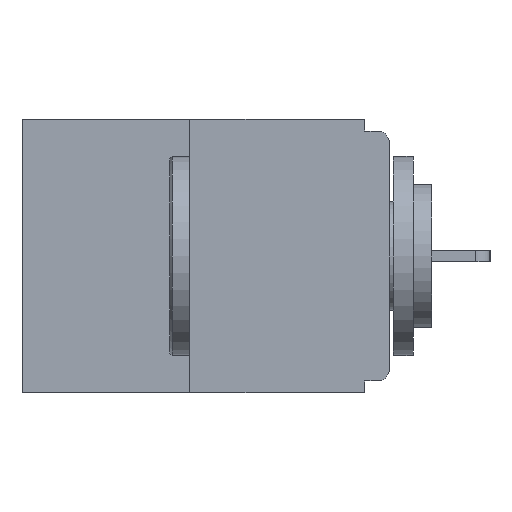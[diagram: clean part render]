
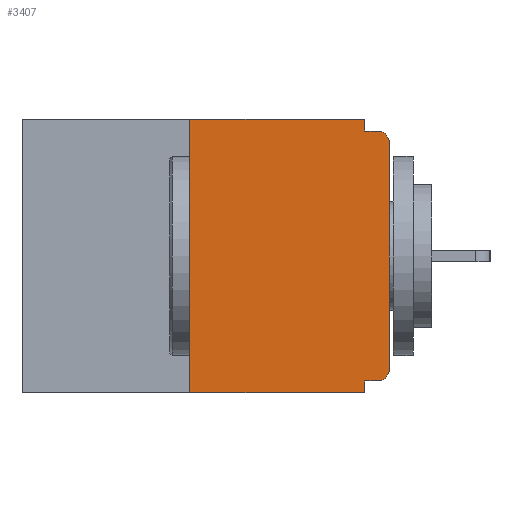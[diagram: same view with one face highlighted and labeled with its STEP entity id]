
A CAD part, left-side view. The second image highlights one B-rep face of the part: STEP entity #3407.
In plain terms, the highlighted planar face has unit normal (-1, 0, 0).
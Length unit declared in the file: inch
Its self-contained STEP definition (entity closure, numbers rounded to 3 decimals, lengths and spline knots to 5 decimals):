
#260 = VERTEX_POINT ( 'NONE', #3799 ) ;
#316 = CARTESIAN_POINT ( 'NONE',  ( 0., 0., 0. ) ) ;
#791 = AXIS2_PLACEMENT_3D ( 'NONE', #11645, #15916, #11462 ) ;
#818 = CARTESIAN_POINT ( 'NONE',  ( 0., 0., -0.03 ) ) ;
#1094 = LINE ( 'NONE', #6852, #12949 ) ;
#1300 = CARTESIAN_POINT ( 'NONE',  ( 0., 0.46, 0. ) ) ;
#1561 = DIRECTION ( 'NONE',  ( 0., 1., 0. ) ) ;
#1620 = VERTEX_POINT ( 'NONE', #3096 ) ;
#1744 = ORIENTED_EDGE ( 'NONE', *, *, #5236, .F. ) ;
#1764 = EDGE_CURVE ( 'NONE', #12057, #2645, #15228, .T. ) ;
#1953 = CARTESIAN_POINT ( 'NONE',  ( 0., 0.031, -0.328 ) ) ;
#2507 = VECTOR ( 'NONE', #6049, 39.37008 ) ;
#2645 = VERTEX_POINT ( 'NONE', #7402 ) ;
#3096 = CARTESIAN_POINT ( 'NONE',  ( 0., 0.25, -0.343 ) ) ;
#3197 = CIRCLE ( 'NONE', #6806, 0.015 ) ;
#3407 = ADVANCED_FACE ( 'NONE', ( #15350 ), #7149, .F. ) ;
#3560 = DIRECTION ( 'NONE',  ( 0., -1., 0. ) ) ;
#3799 = CARTESIAN_POINT ( 'NONE',  ( 0., 0.015, -0.328 ) ) ;
#3815 = AXIS2_PLACEMENT_3D ( 'NONE', #1300, #11373, #11275 ) ;
#3938 = VECTOR ( 'NONE', #10862, 39.37008 ) ;
#4497 = LINE ( 'NONE', #15814, #15665 ) ;
#4997 = ORIENTED_EDGE ( 'NONE', *, *, #9767, .T. ) ;
#5148 = CARTESIAN_POINT ( 'NONE',  ( 0., 0., -0.015 ) ) ;
#5236 = EDGE_CURVE ( 'NONE', #14864, #13512, #17326, .T. ) ;
#5780 = DIRECTION ( 'NONE',  ( 0., -1., 0. ) ) ;
#5905 = CARTESIAN_POINT ( 'NONE',  ( 0., 0.031, -0.343 ) ) ;
#6049 = DIRECTION ( 'NONE',  ( 0., 0., 1. ) ) ;
#6182 = DIRECTION ( 'NONE',  ( 0., 0., 1. ) ) ;
#6338 = ORIENTED_EDGE ( 'NONE', *, *, #9928, .T. ) ;
#6625 = EDGE_CURVE ( 'NONE', #11331, #8140, #8690, .T. ) ;
#6680 = CARTESIAN_POINT ( 'NONE',  ( 0., 0.015, -0.03 ) ) ;
#6690 = EDGE_CURVE ( 'NONE', #9178, #13373, #7468, .T. ) ;
#6806 = AXIS2_PLACEMENT_3D ( 'NONE', #6680, #9854, #13861 ) ;
#6852 = CARTESIAN_POINT ( 'NONE',  ( 0., 0.46, -0.343 ) ) ;
#7149 = PLANE ( 'NONE',  #3815 ) ;
#7188 = CARTESIAN_POINT ( 'NONE',  ( 0., 0.46, 0. ) ) ;
#7373 = EDGE_CURVE ( 'NONE', #260, #14864, #13103, .T. ) ;
#7402 = CARTESIAN_POINT ( 'NONE',  ( 0., 0.015, -0.015 ) ) ;
#7468 = LINE ( 'NONE', #316, #2507 ) ;
#7970 = CARTESIAN_POINT ( 'NONE',  ( 0., 0.031, -0.015 ) ) ;
#8140 = VERTEX_POINT ( 'NONE', #11102 ) ;
#8673 = CARTESIAN_POINT ( 'NONE',  ( 0., 0.25, 0. ) ) ;
#8690 = LINE ( 'NONE', #7188, #9167 ) ;
#8768 = ORIENTED_EDGE ( 'NONE', *, *, #6690, .T. ) ;
#9167 = VECTOR ( 'NONE', #5780, 39.37008 ) ;
#9178 = VERTEX_POINT ( 'NONE', #17644 ) ;
#9519 = ORIENTED_EDGE ( 'NONE', *, *, #6625, .F. ) ;
#9767 = EDGE_CURVE ( 'NONE', #13373, #2645, #3197, .T. ) ;
#9854 = DIRECTION ( 'NONE',  ( -1., 0., 0. ) ) ;
#9928 = EDGE_CURVE ( 'NONE', #260, #9178, #12185, .T. ) ;
#9982 = ORIENTED_EDGE ( 'NONE', *, *, #16427, .F. ) ;
#10029 = VECTOR ( 'NONE', #1561, 39.37008 ) ;
#10482 = CARTESIAN_POINT ( 'NONE',  ( 0., 0., -0.328 ) ) ;
#10495 = DIRECTION ( 'NONE',  ( 0., 0., -1. ) ) ;
#10521 = EDGE_CURVE ( 'NONE', #8140, #12057, #16958, .T. ) ;
#10833 = ORIENTED_EDGE ( 'NONE', *, *, #13390, .T. ) ;
#10862 = DIRECTION ( 'NONE',  ( 0., -1., 0. ) ) ;
#11102 = CARTESIAN_POINT ( 'NONE',  ( 0., 0.031, 0. ) ) ;
#11168 = DIRECTION ( 'NONE',  ( 0., 0., -1. ) ) ;
#11275 = DIRECTION ( 'NONE',  ( 0., 0., -1. ) ) ;
#11331 = VERTEX_POINT ( 'NONE', #8673 ) ;
#11373 = DIRECTION ( 'NONE',  ( 1., 0., 0. ) ) ;
#11462 = DIRECTION ( 'NONE',  ( 0., 0., -1. ) ) ;
#11553 = CARTESIAN_POINT ( 'NONE',  ( 0., 0.031, 0. ) ) ;
#11645 = CARTESIAN_POINT ( 'NONE',  ( 0., 0.015, -0.313 ) ) ;
#12057 = VERTEX_POINT ( 'NONE', #7970 ) ;
#12185 = CIRCLE ( 'NONE', #791, 0.015 ) ;
#12949 = VECTOR ( 'NONE', #3560, 39.37008 ) ;
#13103 = LINE ( 'NONE', #10482, #10029 ) ;
#13373 = VERTEX_POINT ( 'NONE', #818 ) ;
#13390 = EDGE_CURVE ( 'NONE', #1620, #13512, #1094, .T. ) ;
#13512 = VERTEX_POINT ( 'NONE', #5905 ) ;
#13646 = EDGE_LOOP ( 'NONE', ( #9519, #9982, #10833, #1744, #17591, #6338, #8768, #4997, #14006, #16233 ) ) ;
#13861 = DIRECTION ( 'NONE',  ( 0., 0., -1. ) ) ;
#14006 = ORIENTED_EDGE ( 'NONE', *, *, #1764, .F. ) ;
#14682 = CARTESIAN_POINT ( 'NONE',  ( 0., 0.031, -0.343 ) ) ;
#14864 = VERTEX_POINT ( 'NONE', #1953 ) ;
#15228 = LINE ( 'NONE', #5148, #3938 ) ;
#15350 = FACE_OUTER_BOUND ( 'NONE', #13646, .T. ) ;
#15665 = VECTOR ( 'NONE', #6182, 39.37008 ) ;
#15814 = CARTESIAN_POINT ( 'NONE',  ( 0., 0.25, 0. ) ) ;
#15822 = VECTOR ( 'NONE', #10495, 39.37008 ) ;
#15916 = DIRECTION ( 'NONE',  ( -1., 0., 0. ) ) ;
#16233 = ORIENTED_EDGE ( 'NONE', *, *, #10521, .F. ) ;
#16427 = EDGE_CURVE ( 'NONE', #1620, #11331, #4497, .T. ) ;
#16958 = LINE ( 'NONE', #11553, #17873 ) ;
#17326 = LINE ( 'NONE', #14682, #15822 ) ;
#17591 = ORIENTED_EDGE ( 'NONE', *, *, #7373, .F. ) ;
#17644 = CARTESIAN_POINT ( 'NONE',  ( 0., 0., -0.313 ) ) ;
#17873 = VECTOR ( 'NONE', #11168, 39.37008 ) ;
